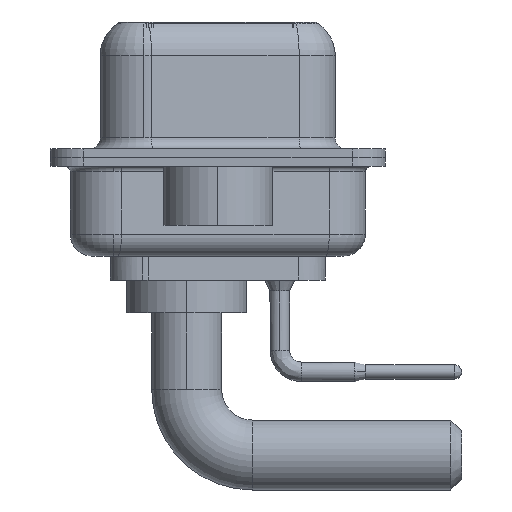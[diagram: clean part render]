
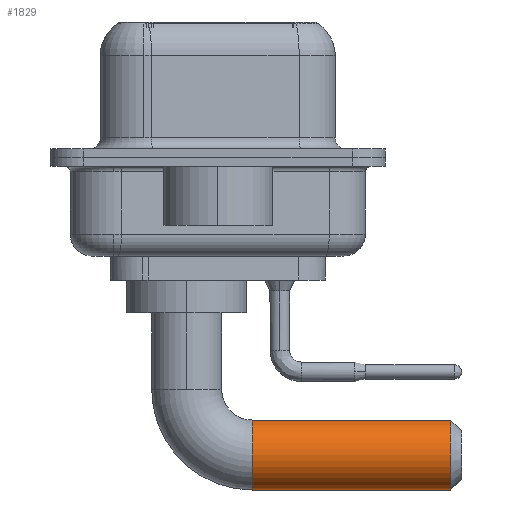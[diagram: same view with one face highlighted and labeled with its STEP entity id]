
A CAD part, left-side view. The second image highlights one B-rep face of the part: STEP entity #1829.
In plain terms, the highlighted cylindrical face has radius 1.6 mm (diameter 3.2 mm), a partial arc.
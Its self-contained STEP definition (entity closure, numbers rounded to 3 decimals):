
#811 = ORIENTED_EDGE ( 'NONE', *, *, #14070, .T. ) ;
#1718 = EDGE_CURVE ( 'NONE', #6967, #6596, #12760, .T. ) ;
#1829 = ADVANCED_FACE ( 'NONE', ( #12631 ), #9416, .T. ) ;
#2625 = DIRECTION ( 'NONE',  ( 0., 0., -1. ) ) ;
#2940 = DIRECTION ( 'NONE',  ( 0., 1., 0. ) ) ;
#3734 = VERTEX_POINT ( 'NONE', #17375 ) ;
#4126 = CARTESIAN_POINT ( 'NONE',  ( 0., -3., -4.9 ) ) ;
#4559 = ORIENTED_EDGE ( 'NONE', *, *, #10906, .T. ) ;
#4641 = DIRECTION ( 'NONE',  ( 0., -1., 0. ) ) ;
#5601 = CARTESIAN_POINT ( 'NONE',  ( 0., -3., -8.1 ) ) ;
#5982 = CIRCLE ( 'NONE', #10077, 1.6 ) ;
#6596 = VERTEX_POINT ( 'NONE', #13994 ) ;
#6967 = VERTEX_POINT ( 'NONE', #4126 ) ;
#7317 = LINE ( 'NONE', #5601, #19346 ) ;
#7604 = DIRECTION ( 'NONE',  ( 0., 0., -1. ) ) ;
#7829 = CARTESIAN_POINT ( 'NONE',  ( 0., -3., -6.5 ) ) ;
#8953 = DIRECTION ( 'NONE',  ( 0., -1., 0. ) ) ;
#9416 = CYLINDRICAL_SURFACE ( 'NONE', #13512, 1.6 ) ;
#9723 = ORIENTED_EDGE ( 'NONE', *, *, #1718, .F. ) ;
#10077 = AXIS2_PLACEMENT_3D ( 'NONE', #14379, #2940, #2625 ) ;
#10123 = VECTOR ( 'NONE', #4641, 1000. ) ;
#10147 = ORIENTED_EDGE ( 'NONE', *, *, #12748, .T. ) ;
#10906 = EDGE_CURVE ( 'NONE', #6967, #12139, #18629, .T. ) ;
#12139 = VERTEX_POINT ( 'NONE', #18093 ) ;
#12631 = FACE_OUTER_BOUND ( 'NONE', #17933, .T. ) ;
#12748 = EDGE_CURVE ( 'NONE', #12139, #3734, #7317, .T. ) ;
#12760 = LINE ( 'NONE', #17801, #10123 ) ;
#13512 = AXIS2_PLACEMENT_3D ( 'NONE', #7829, #20640, #7604 ) ;
#13994 = CARTESIAN_POINT ( 'NONE',  ( 0., -12.07, -4.9 ) ) ;
#14070 = EDGE_CURVE ( 'NONE', #3734, #6596, #5982, .T. ) ;
#14379 = CARTESIAN_POINT ( 'NONE',  ( 0., -12.07, -6.5 ) ) ;
#15256 = CARTESIAN_POINT ( 'NONE',  ( 0., -3., -6.5 ) ) ;
#15457 = DIRECTION ( 'NONE',  ( -1., 0., 0. ) ) ;
#16674 = DIRECTION ( 'NONE',  ( 0., -1., 0. ) ) ;
#17375 = CARTESIAN_POINT ( 'NONE',  ( 0., -12.07, -8.1 ) ) ;
#17801 = CARTESIAN_POINT ( 'NONE',  ( 0., -3., -4.9 ) ) ;
#17933 = EDGE_LOOP ( 'NONE', ( #9723, #4559, #10147, #811 ) ) ;
#18093 = CARTESIAN_POINT ( 'NONE',  ( 0., -3., -8.1 ) ) ;
#18629 = CIRCLE ( 'NONE', #19666, 1.6 ) ;
#19346 = VECTOR ( 'NONE', #16674, 1000. ) ;
#19666 = AXIS2_PLACEMENT_3D ( 'NONE', #15256, #8953, #15457 ) ;
#20640 = DIRECTION ( 'NONE',  ( 0., -1., 0. ) ) ;
